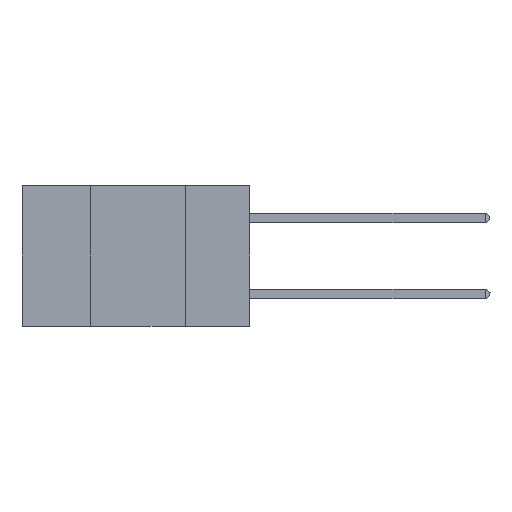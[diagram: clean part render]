
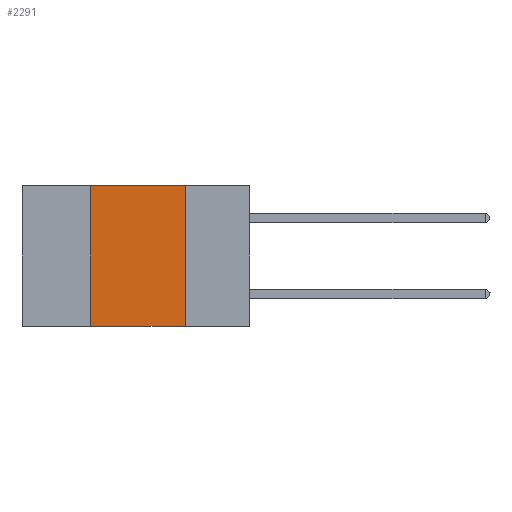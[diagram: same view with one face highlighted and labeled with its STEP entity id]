
A CAD part, left-side view. The second image highlights one B-rep face of the part: STEP entity #2291.
In plain terms, the highlighted planar face has unit normal (-1, 0, 0).
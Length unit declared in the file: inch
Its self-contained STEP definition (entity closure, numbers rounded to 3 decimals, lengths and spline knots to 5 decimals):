
#492 = CARTESIAN_POINT ( 'NONE',  ( 0., 0.17, -0.37 ) ) ;
#686 = VECTOR ( 'NONE', #10138, 39.37008 ) ;
#1158 = EDGE_CURVE ( 'NONE', #4518, #11016, #1902, .T. ) ;
#1161 = EDGE_CURVE ( 'NONE', #11016, #2966, #7039, .T. ) ;
#1902 = LINE ( 'NONE', #7980, #8100 ) ;
#2291 = ADVANCED_FACE ( 'NONE', ( #9555 ), #11175, .F. ) ;
#2966 = VERTEX_POINT ( 'NONE', #492 ) ;
#3010 = EDGE_CURVE ( 'NONE', #4810, #4518, #7380, .T. ) ;
#3163 = AXIS2_PLACEMENT_3D ( 'NONE', #10462, #6830, #10354 ) ;
#4046 = CARTESIAN_POINT ( 'NONE',  ( 0., 0.42, 0. ) ) ;
#4276 = ORIENTED_EDGE ( 'NONE', *, *, #3010, .F. ) ;
#4281 = DIRECTION ( 'NONE',  ( 0., 0., -1. ) ) ;
#4513 = CARTESIAN_POINT ( 'NONE',  ( 0., 0.17, 0. ) ) ;
#4518 = VERTEX_POINT ( 'NONE', #4046 ) ;
#4810 = VERTEX_POINT ( 'NONE', #5799 ) ;
#5799 = CARTESIAN_POINT ( 'NONE',  ( 0., 0.42, -0.37 ) ) ;
#6067 = DIRECTION ( 'NONE',  ( 0., -1., 0. ) ) ;
#6105 = ORIENTED_EDGE ( 'NONE', *, *, #10148, .T. ) ;
#6830 = DIRECTION ( 'NONE',  ( 1., 0., 0. ) ) ;
#7000 = ORIENTED_EDGE ( 'NONE', *, *, #1161, .F. ) ;
#7039 = LINE ( 'NONE', #4513, #8279 ) ;
#7177 = EDGE_LOOP ( 'NONE', ( #7000, #8581, #4276, #6105 ) ) ;
#7380 = LINE ( 'NONE', #10144, #9078 ) ;
#7543 = LINE ( 'NONE', #8572, #686 ) ;
#7786 = CARTESIAN_POINT ( 'NONE',  ( 0., 0.17, 0. ) ) ;
#7980 = CARTESIAN_POINT ( 'NONE',  ( 0., 0.6, 0. ) ) ;
#8100 = VECTOR ( 'NONE', #6067, 39.37008 ) ;
#8279 = VECTOR ( 'NONE', #4281, 39.37008 ) ;
#8572 = CARTESIAN_POINT ( 'NONE',  ( 0., 0.6, -0.37 ) ) ;
#8581 = ORIENTED_EDGE ( 'NONE', *, *, #1158, .F. ) ;
#9078 = VECTOR ( 'NONE', #11015, 39.37008 ) ;
#9555 = FACE_OUTER_BOUND ( 'NONE', #7177, .T. ) ;
#10138 = DIRECTION ( 'NONE',  ( 0., -1., 0. ) ) ;
#10144 = CARTESIAN_POINT ( 'NONE',  ( 0., 0.42, 0. ) ) ;
#10148 = EDGE_CURVE ( 'NONE', #4810, #2966, #7543, .T. ) ;
#10354 = DIRECTION ( 'NONE',  ( 0., 0., -1. ) ) ;
#10462 = CARTESIAN_POINT ( 'NONE',  ( 0., 0.6, 0. ) ) ;
#11015 = DIRECTION ( 'NONE',  ( 0., 0., 1. ) ) ;
#11016 = VERTEX_POINT ( 'NONE', #7786 ) ;
#11175 = PLANE ( 'NONE',  #3163 ) ;
